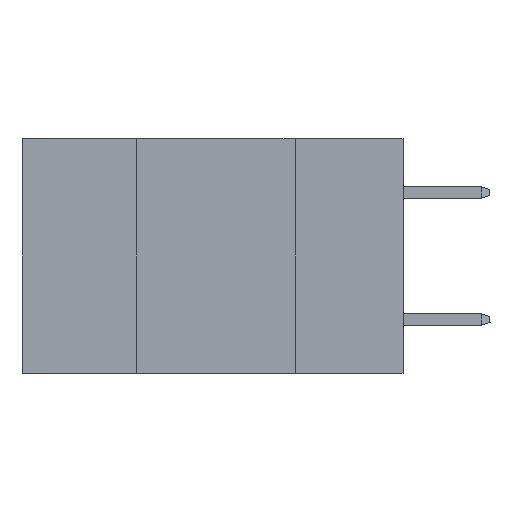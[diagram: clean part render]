
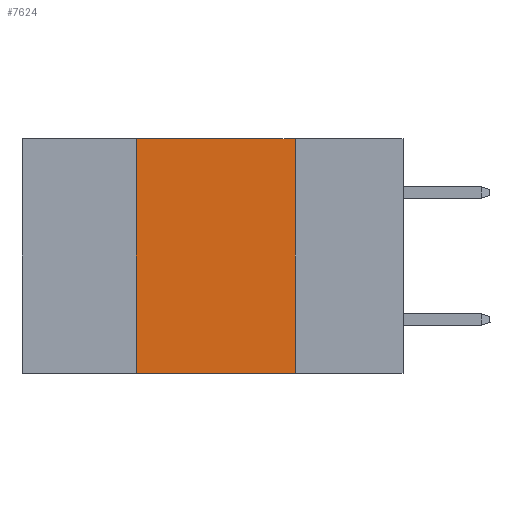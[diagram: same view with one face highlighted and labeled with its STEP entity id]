
A CAD part, left-side view. The second image highlights one B-rep face of the part: STEP entity #7624.
In plain terms, the highlighted planar face has unit normal (-1, 0, 0).
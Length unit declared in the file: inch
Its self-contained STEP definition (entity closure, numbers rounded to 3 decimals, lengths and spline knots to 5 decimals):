
#11 = VECTOR ( 'NONE', #8262, 39.37008 ) ;
#610 = CARTESIAN_POINT ( 'NONE',  ( 0., 0.42, 0. ) ) ;
#1008 = CARTESIAN_POINT ( 'NONE',  ( 0., 0.17, 0. ) ) ;
#1532 = VERTEX_POINT ( 'NONE', #17638 ) ;
#2094 = EDGE_CURVE ( 'NONE', #12024, #22280, #7391, .T. ) ;
#2579 = EDGE_CURVE ( 'NONE', #20686, #1532, #15385, .T. ) ;
#4050 = DIRECTION ( 'NONE',  ( 0., 0., 1. ) ) ;
#4504 = CARTESIAN_POINT ( 'NONE',  ( 0., 0.6, 0. ) ) ;
#4540 = ORIENTED_EDGE ( 'NONE', *, *, #20980, .F. ) ;
#5361 = CARTESIAN_POINT ( 'NONE',  ( 0., 0.42, 0. ) ) ;
#6543 = VECTOR ( 'NONE', #16988, 39.37008 ) ;
#7391 = LINE ( 'NONE', #5361, #23041 ) ;
#7624 = ADVANCED_FACE ( 'NONE', ( #11901 ), #11423, .F. ) ;
#7818 = EDGE_LOOP ( 'NONE', ( #16465, #4540, #12601, #14121 ) ) ;
#8262 = DIRECTION ( 'NONE',  ( 0., 0., -1. ) ) ;
#11342 = LINE ( 'NONE', #13475, #11952 ) ;
#11423 = PLANE ( 'NONE',  #11445 ) ;
#11445 = AXIS2_PLACEMENT_3D ( 'NONE', #17107, #13440, #19120 ) ;
#11901 = FACE_OUTER_BOUND ( 'NONE', #7818, .T. ) ;
#11952 = VECTOR ( 'NONE', #20680, 39.37008 ) ;
#12024 = VERTEX_POINT ( 'NONE', #15968 ) ;
#12601 = ORIENTED_EDGE ( 'NONE', *, *, #2094, .F. ) ;
#13440 = DIRECTION ( 'NONE',  ( 1., 0., 0. ) ) ;
#13475 = CARTESIAN_POINT ( 'NONE',  ( 0., 0.6, -0.37 ) ) ;
#14121 = ORIENTED_EDGE ( 'NONE', *, *, #16717, .T. ) ;
#14134 = LINE ( 'NONE', #4504, #6543 ) ;
#15385 = LINE ( 'NONE', #1008, #11 ) ;
#15583 = CARTESIAN_POINT ( 'NONE',  ( 0., 0.17, 0. ) ) ;
#15968 = CARTESIAN_POINT ( 'NONE',  ( 0., 0.42, -0.37 ) ) ;
#16465 = ORIENTED_EDGE ( 'NONE', *, *, #2579, .F. ) ;
#16717 = EDGE_CURVE ( 'NONE', #12024, #1532, #11342, .T. ) ;
#16988 = DIRECTION ( 'NONE',  ( 0., -1., 0. ) ) ;
#17107 = CARTESIAN_POINT ( 'NONE',  ( 0., 0.6, 0. ) ) ;
#17638 = CARTESIAN_POINT ( 'NONE',  ( 0., 0.17, -0.37 ) ) ;
#19120 = DIRECTION ( 'NONE',  ( 0., 0., -1. ) ) ;
#20680 = DIRECTION ( 'NONE',  ( 0., -1., 0. ) ) ;
#20686 = VERTEX_POINT ( 'NONE', #15583 ) ;
#20980 = EDGE_CURVE ( 'NONE', #22280, #20686, #14134, .T. ) ;
#22280 = VERTEX_POINT ( 'NONE', #610 ) ;
#23041 = VECTOR ( 'NONE', #4050, 39.37008 ) ;
